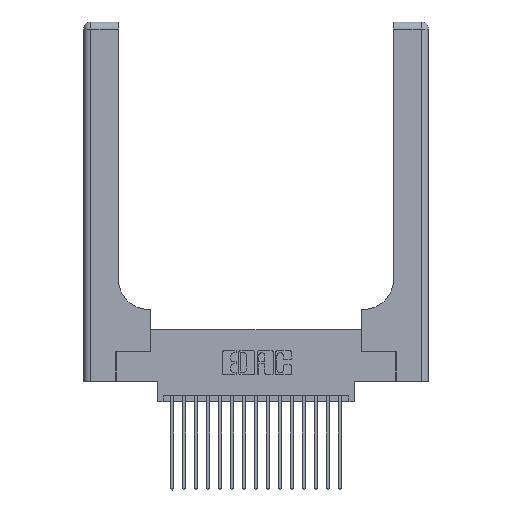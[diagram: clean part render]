
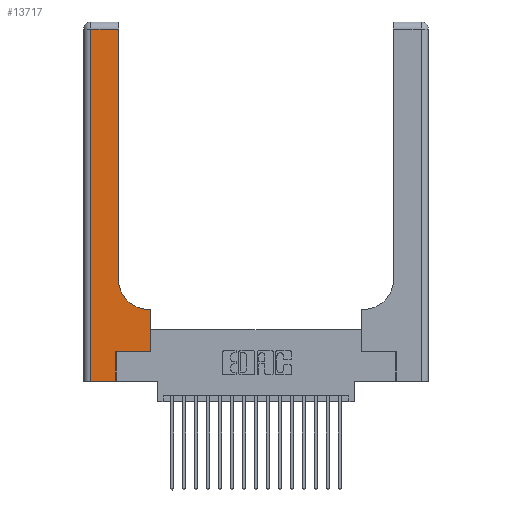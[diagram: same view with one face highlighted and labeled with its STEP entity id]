
A CAD part, top view. The second image highlights one B-rep face of the part: STEP entity #13717.
In plain terms, the highlighted planar face has unit normal (0, 0, 1).
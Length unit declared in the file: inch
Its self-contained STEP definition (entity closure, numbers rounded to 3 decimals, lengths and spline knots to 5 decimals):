
#402 = EDGE_CURVE ( 'NONE', #15682, #5852, #4415, .T. ) ;
#686 = VERTEX_POINT ( 'NONE', #4694 ) ;
#873 = LINE ( 'NONE', #1547, #12924 ) ;
#915 = VERTEX_POINT ( 'NONE', #11134 ) ;
#1061 = ORIENTED_EDGE ( 'NONE', *, *, #402, .T. ) ;
#1077 = VERTEX_POINT ( 'NONE', #6681 ) ;
#1402 = EDGE_CURVE ( 'NONE', #5852, #686, #16954, .T. ) ;
#1547 = CARTESIAN_POINT ( 'NONE',  ( 0.2915, 3., 0.37 ) ) ;
#2227 = CARTESIAN_POINT ( 'NONE',  ( 0., 0., 0.37 ) ) ;
#2390 = VECTOR ( 'NONE', #16773, 39.37008 ) ;
#3162 = DIRECTION ( 'NONE',  ( 0., 1., 0. ) ) ;
#4231 = AXIS2_PLACEMENT_3D ( 'NONE', #8499, #5270, #10019 ) ;
#4343 = VECTOR ( 'NONE', #6956, 39.37008 ) ;
#4415 = LINE ( 'NONE', #2227, #2390 ) ;
#4694 = CARTESIAN_POINT ( 'NONE',  ( 0.269, 0.25, 0.37 ) ) ;
#4729 = EDGE_CURVE ( 'NONE', #8126, #1077, #10783, .T. ) ;
#5141 = VECTOR ( 'NONE', #17116, 39.37008 ) ;
#5270 = DIRECTION ( 'NONE',  ( 0., 0., -1. ) ) ;
#5852 = VERTEX_POINT ( 'NONE', #18605 ) ;
#6467 = DIRECTION ( 'NONE',  ( 0., -1., 0. ) ) ;
#6634 = DIRECTION ( 'NONE',  ( 0., 1., 0. ) ) ;
#6681 = CARTESIAN_POINT ( 'NONE',  ( 0.5585, 0.6, 0.37 ) ) ;
#6803 = ORIENTED_EDGE ( 'NONE', *, *, #19756, .T. ) ;
#6830 = ORIENTED_EDGE ( 'NONE', *, *, #7972, .T. ) ;
#6956 = DIRECTION ( 'NONE',  ( -1., 0., 0. ) ) ;
#7491 = ORIENTED_EDGE ( 'NONE', *, *, #9486, .T. ) ;
#7972 = EDGE_CURVE ( 'NONE', #686, #8126, #12669, .T. ) ;
#8126 = VERTEX_POINT ( 'NONE', #8128 ) ;
#8128 = CARTESIAN_POINT ( 'NONE',  ( 0.5585, 0.25, 0.37 ) ) ;
#8499 = CARTESIAN_POINT ( 'NONE',  ( 0., 3., 0.37 ) ) ;
#8701 = EDGE_CURVE ( 'NONE', #20162, #12419, #873, .T. ) ;
#8842 = VERTEX_POINT ( 'NONE', #17905 ) ;
#9011 = VECTOR ( 'NONE', #13651, 39.37008 ) ;
#9326 = LINE ( 'NONE', #13519, #14607 ) ;
#9381 = VECTOR ( 'NONE', #6467, 39.37008 ) ;
#9486 = EDGE_CURVE ( 'NONE', #915, #15682, #20164, .T. ) ;
#9655 = EDGE_CURVE ( 'NONE', #12419, #915, #14405, .T. ) ;
#9823 = ORIENTED_EDGE ( 'NONE', *, *, #1402, .T. ) ;
#10019 = DIRECTION ( 'NONE',  ( -1., 0., 0. ) ) ;
#10516 = EDGE_CURVE ( 'NONE', #1077, #8842, #9326, .T. ) ;
#10673 = ORIENTED_EDGE ( 'NONE', *, *, #10516, .T. ) ;
#10783 = LINE ( 'NONE', #12190, #9011 ) ;
#11134 = CARTESIAN_POINT ( 'NONE',  ( 0.06, 2.94, 0.37 ) ) ;
#11149 = CARTESIAN_POINT ( 'NONE',  ( 0.2915, 0.85, 0.37 ) ) ;
#11359 = DIRECTION ( 'NONE',  ( -1., 0., 0. ) ) ;
#11775 = CARTESIAN_POINT ( 'NONE',  ( 0.06, 0., 0.37 ) ) ;
#12190 = CARTESIAN_POINT ( 'NONE',  ( 0.5585, 0.25, 0.37 ) ) ;
#12320 = EDGE_LOOP ( 'NONE', ( #18541, #19750, #7491, #1061, #9823, #6830, #18323, #10673, #6803 ) ) ;
#12419 = VERTEX_POINT ( 'NONE', #20327 ) ;
#12669 = LINE ( 'NONE', #20592, #5141 ) ;
#12814 = CARTESIAN_POINT ( 'NONE',  ( 0.269, 0., 0.37 ) ) ;
#12924 = VECTOR ( 'NONE', #6634, 39.37008 ) ;
#13311 = CARTESIAN_POINT ( 'NONE',  ( 0., 2.94, 0.37 ) ) ;
#13519 = CARTESIAN_POINT ( 'NONE',  ( 0.2915, 0.6, 0.37 ) ) ;
#13651 = DIRECTION ( 'NONE',  ( 0., 1., 0. ) ) ;
#13717 = ADVANCED_FACE ( 'NONE', ( #19725 ), #19627, .F. ) ;
#14405 = LINE ( 'NONE', #13311, #4343 ) ;
#14592 = CARTESIAN_POINT ( 'NONE',  ( 0.06, 3., 0.37 ) ) ;
#14607 = VECTOR ( 'NONE', #11359, 39.37008 ) ;
#14944 = VECTOR ( 'NONE', #3162, 39.37008 ) ;
#15682 = VERTEX_POINT ( 'NONE', #11775 ) ;
#16431 = CARTESIAN_POINT ( 'NONE',  ( 0.5415, 0.85, 0.37 ) ) ;
#16773 = DIRECTION ( 'NONE',  ( 1., 0., 0. ) ) ;
#16954 = LINE ( 'NONE', #12814, #14944 ) ;
#17116 = DIRECTION ( 'NONE',  ( 1., 0., 0. ) ) ;
#17905 = CARTESIAN_POINT ( 'NONE',  ( 0.5415, 0.6, 0.37 ) ) ;
#18028 = DIRECTION ( 'NONE',  ( 1., 0., 0. ) ) ;
#18323 = ORIENTED_EDGE ( 'NONE', *, *, #4729, .T. ) ;
#18446 = CIRCLE ( 'NONE', #20254, 0.25 ) ;
#18541 = ORIENTED_EDGE ( 'NONE', *, *, #8701, .T. ) ;
#18605 = CARTESIAN_POINT ( 'NONE',  ( 0.269, 0., 0.37 ) ) ;
#19627 = PLANE ( 'NONE',  #4231 ) ;
#19633 = DIRECTION ( 'NONE',  ( 0., 0., -1. ) ) ;
#19725 = FACE_OUTER_BOUND ( 'NONE', #12320, .T. ) ;
#19750 = ORIENTED_EDGE ( 'NONE', *, *, #9655, .T. ) ;
#19756 = EDGE_CURVE ( 'NONE', #8842, #20162, #18446, .T. ) ;
#20162 = VERTEX_POINT ( 'NONE', #11149 ) ;
#20164 = LINE ( 'NONE', #14592, #9381 ) ;
#20254 = AXIS2_PLACEMENT_3D ( 'NONE', #16431, #19633, #18028 ) ;
#20327 = CARTESIAN_POINT ( 'NONE',  ( 0.2915, 2.94, 0.37 ) ) ;
#20592 = CARTESIAN_POINT ( 'NONE',  ( 0.269, 0.25, 0.37 ) ) ;
